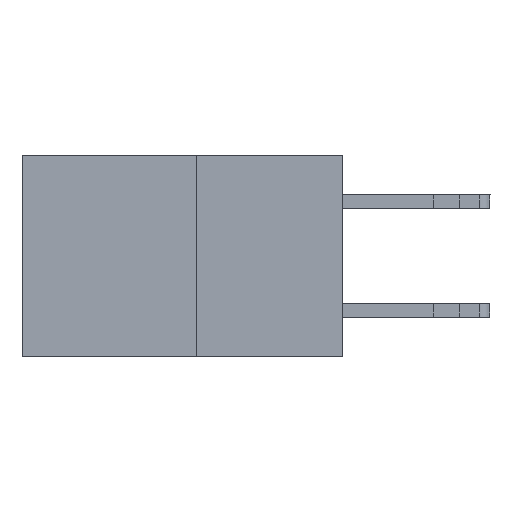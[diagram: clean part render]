
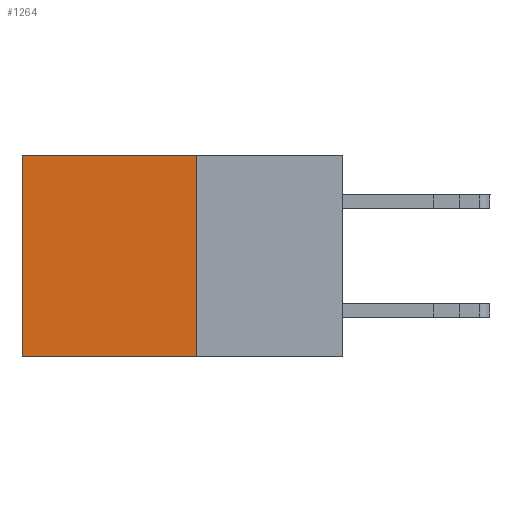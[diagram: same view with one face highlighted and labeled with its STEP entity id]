
A CAD part, left-side view. The second image highlights one B-rep face of the part: STEP entity #1264.
In plain terms, the highlighted planar face has unit normal (-1, 0, 0).
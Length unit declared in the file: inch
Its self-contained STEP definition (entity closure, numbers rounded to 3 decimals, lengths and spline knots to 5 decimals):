
#57 = DIRECTION ( 'NONE',  ( 0., 1., 0. ) ) ;
#572 = VECTOR ( 'NONE', #57, 39.37008 ) ;
#951 = CARTESIAN_POINT ( 'NONE',  ( 0.277, 0.59, -0.37 ) ) ;
#1198 = LINE ( 'NONE', #12428, #18729 ) ;
#1264 = ADVANCED_FACE ( 'NONE', ( #15135 ), #22696, .F. ) ;
#1443 = ORIENTED_EDGE ( 'NONE', *, *, #9510, .F. ) ;
#3697 = CARTESIAN_POINT ( 'NONE',  ( 0.277, 0.27, 0. ) ) ;
#3753 = EDGE_CURVE ( 'NONE', #19855, #14891, #13104, .T. ) ;
#4768 = DIRECTION ( 'NONE',  ( 0., 0., -1. ) ) ;
#7600 = EDGE_LOOP ( 'NONE', ( #19505, #23210, #1443, #21254 ) ) ;
#7656 = DIRECTION ( 'NONE',  ( 1., 0., 0. ) ) ;
#8546 = DIRECTION ( 'NONE',  ( 0., 1., 0. ) ) ;
#9473 = VECTOR ( 'NONE', #4768, 39.37008 ) ;
#9510 = EDGE_CURVE ( 'NONE', #17823, #19855, #1198, .T. ) ;
#10467 = CARTESIAN_POINT ( 'NONE',  ( 0.277, 0.59, 0. ) ) ;
#12428 = CARTESIAN_POINT ( 'NONE',  ( 0.277, 0.27, -0.37 ) ) ;
#12496 = LINE ( 'NONE', #23458, #9473 ) ;
#13092 = DIRECTION ( 'NONE',  ( 0., 0., -1. ) ) ;
#13104 = LINE ( 'NONE', #20879, #572 ) ;
#13210 = VERTEX_POINT ( 'NONE', #10467 ) ;
#13697 = EDGE_CURVE ( 'NONE', #13210, #14891, #12496, .T. ) ;
#14891 = VERTEX_POINT ( 'NONE', #951 ) ;
#15135 = FACE_OUTER_BOUND ( 'NONE', #7600, .T. ) ;
#16285 = CARTESIAN_POINT ( 'NONE',  ( 0.277, 0.27, 0. ) ) ;
#16373 = CARTESIAN_POINT ( 'NONE',  ( 0.277, 0.27, -0.37 ) ) ;
#17823 = VERTEX_POINT ( 'NONE', #3697 ) ;
#18729 = VECTOR ( 'NONE', #21552, 39.37008 ) ;
#19505 = ORIENTED_EDGE ( 'NONE', *, *, #13697, .T. ) ;
#19690 = AXIS2_PLACEMENT_3D ( 'NONE', #22563, #7656, #13092 ) ;
#19855 = VERTEX_POINT ( 'NONE', #16373 ) ;
#19941 = LINE ( 'NONE', #16285, #21876 ) ;
#20879 = CARTESIAN_POINT ( 'NONE',  ( 0.277, 0.27, -0.37 ) ) ;
#21254 = ORIENTED_EDGE ( 'NONE', *, *, #21317, .T. ) ;
#21317 = EDGE_CURVE ( 'NONE', #17823, #13210, #19941, .T. ) ;
#21552 = DIRECTION ( 'NONE',  ( 0., 0., -1. ) ) ;
#21876 = VECTOR ( 'NONE', #8546, 39.37008 ) ;
#22563 = CARTESIAN_POINT ( 'NONE',  ( 0.277, 0.27, -0.37 ) ) ;
#22696 = PLANE ( 'NONE',  #19690 ) ;
#23210 = ORIENTED_EDGE ( 'NONE', *, *, #3753, .F. ) ;
#23458 = CARTESIAN_POINT ( 'NONE',  ( 0.277, 0.59, -0.37 ) ) ;
